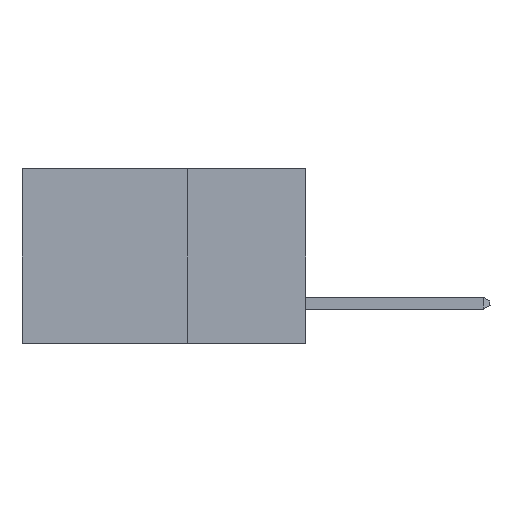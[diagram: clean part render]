
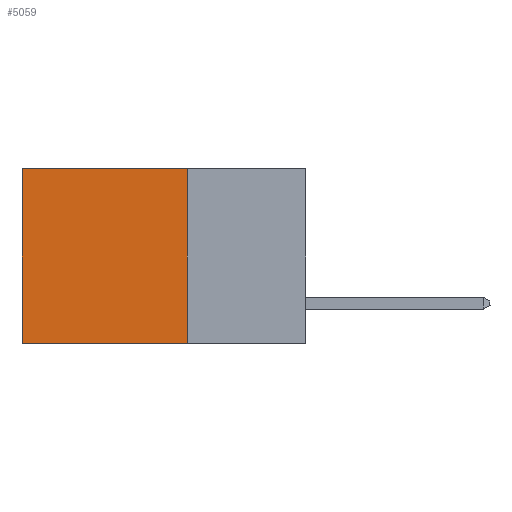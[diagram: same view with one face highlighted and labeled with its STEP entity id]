
A CAD part, left-side view. The second image highlights one B-rep face of the part: STEP entity #5059.
In plain terms, the highlighted planar face has unit normal (-1, 0, 0).
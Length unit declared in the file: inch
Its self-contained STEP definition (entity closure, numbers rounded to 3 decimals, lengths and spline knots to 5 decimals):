
#205 = VECTOR ( 'NONE', #4607, 39.37008 ) ;
#646 = CARTESIAN_POINT ( 'NONE',  ( 0.2615, 0.25, -0.37 ) ) ;
#799 = FACE_OUTER_BOUND ( 'NONE', #3489, .T. ) ;
#1298 = CARTESIAN_POINT ( 'NONE',  ( 0.2615, 0.6, 0. ) ) ;
#2270 = EDGE_CURVE ( 'NONE', #3013, #7467, #5391, .T. ) ;
#2443 = CARTESIAN_POINT ( 'NONE',  ( 0.2615, 0.6, -0.37 ) ) ;
#2450 = EDGE_CURVE ( 'NONE', #11207, #7491, #5714, .T. ) ;
#2949 = AXIS2_PLACEMENT_3D ( 'NONE', #3643, #13981, #11605 ) ;
#3013 = VERTEX_POINT ( 'NONE', #8811 ) ;
#3258 = DIRECTION ( 'NONE',  ( 0., 0., -1. ) ) ;
#3489 = EDGE_LOOP ( 'NONE', ( #10377, #4270, #13190, #10776 ) ) ;
#3643 = CARTESIAN_POINT ( 'NONE',  ( 0.2615, 0.25, -0.37 ) ) ;
#4114 = LINE ( 'NONE', #8765, #5530 ) ;
#4270 = ORIENTED_EDGE ( 'NONE', *, *, #2450, .F. ) ;
#4607 = DIRECTION ( 'NONE',  ( 0., 1., 0. ) ) ;
#5059 = ADVANCED_FACE ( 'NONE', ( #799 ), #10451, .F. ) ;
#5391 = LINE ( 'NONE', #5672, #9117 ) ;
#5530 = VECTOR ( 'NONE', #3258, 39.37008 ) ;
#5672 = CARTESIAN_POINT ( 'NONE',  ( 0.2615, 0.25, 0. ) ) ;
#5714 = LINE ( 'NONE', #11653, #205 ) ;
#5863 = DIRECTION ( 'NONE',  ( 0., 1., 0. ) ) ;
#6636 = EDGE_CURVE ( 'NONE', #7467, #7491, #4114, .T. ) ;
#7374 = DIRECTION ( 'NONE',  ( 0., 0., -1. ) ) ;
#7467 = VERTEX_POINT ( 'NONE', #1298 ) ;
#7491 = VERTEX_POINT ( 'NONE', #2443 ) ;
#8765 = CARTESIAN_POINT ( 'NONE',  ( 0.2615, 0.6, -0.37 ) ) ;
#8811 = CARTESIAN_POINT ( 'NONE',  ( 0.2615, 0.25, 0. ) ) ;
#9117 = VECTOR ( 'NONE', #5863, 39.37008 ) ;
#10377 = ORIENTED_EDGE ( 'NONE', *, *, #6636, .T. ) ;
#10451 = PLANE ( 'NONE',  #2949 ) ;
#10776 = ORIENTED_EDGE ( 'NONE', *, *, #2270, .T. ) ;
#11207 = VERTEX_POINT ( 'NONE', #11709 ) ;
#11605 = DIRECTION ( 'NONE',  ( 0., 0., -1. ) ) ;
#11653 = CARTESIAN_POINT ( 'NONE',  ( 0.2615, 0.25, -0.37 ) ) ;
#11709 = CARTESIAN_POINT ( 'NONE',  ( 0.2615, 0.25, -0.37 ) ) ;
#12261 = LINE ( 'NONE', #646, #14444 ) ;
#12569 = EDGE_CURVE ( 'NONE', #3013, #11207, #12261, .T. ) ;
#13190 = ORIENTED_EDGE ( 'NONE', *, *, #12569, .F. ) ;
#13981 = DIRECTION ( 'NONE',  ( 1., 0., 0. ) ) ;
#14444 = VECTOR ( 'NONE', #7374, 39.37008 ) ;
